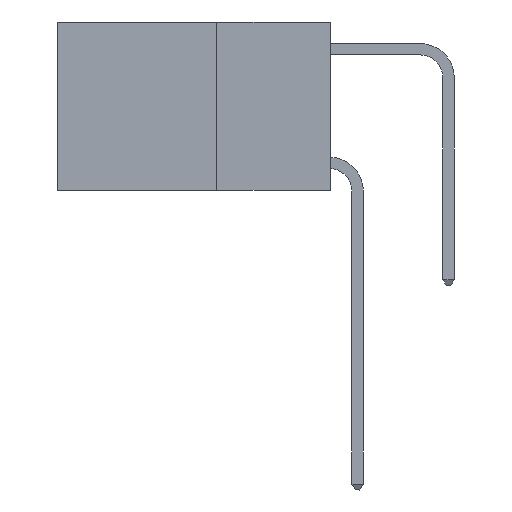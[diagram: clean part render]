
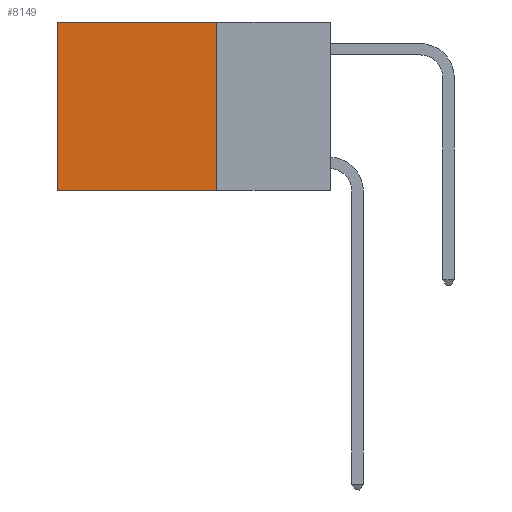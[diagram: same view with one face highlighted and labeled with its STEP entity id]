
A CAD part, left-side view. The second image highlights one B-rep face of the part: STEP entity #8149.
In plain terms, the highlighted planar face has unit normal (-1, 0, 0).
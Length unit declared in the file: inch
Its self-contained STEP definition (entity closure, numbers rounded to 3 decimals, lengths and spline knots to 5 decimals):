
#208 = CARTESIAN_POINT ( 'NONE',  ( 0.2625, 0.25, -0.37 ) ) ;
#336 = CARTESIAN_POINT ( 'NONE',  ( 0.2625, 0.25, 0. ) ) ;
#380 = EDGE_LOOP ( 'NONE', ( #4517, #14074, #3040, #14092 ) ) ;
#546 = DIRECTION ( 'NONE',  ( 0., 0., -1. ) ) ;
#625 = LINE ( 'NONE', #14130, #2360 ) ;
#1012 = VERTEX_POINT ( 'NONE', #6513 ) ;
#2041 = DIRECTION ( 'NONE',  ( 0., 1., 0. ) ) ;
#2360 = VECTOR ( 'NONE', #10369, 39.37008 ) ;
#3040 = ORIENTED_EDGE ( 'NONE', *, *, #4638, .F. ) ;
#3182 = VERTEX_POINT ( 'NONE', #15724 ) ;
#3628 = VECTOR ( 'NONE', #2041, 39.37008 ) ;
#4517 = ORIENTED_EDGE ( 'NONE', *, *, #12804, .T. ) ;
#4638 = EDGE_CURVE ( 'NONE', #3182, #1012, #11636, .T. ) ;
#5042 = LINE ( 'NONE', #208, #11948 ) ;
#5520 = DIRECTION ( 'NONE',  ( 1., 0., 0. ) ) ;
#6513 = CARTESIAN_POINT ( 'NONE',  ( 0.2625, 0.25, -0.37 ) ) ;
#6858 = CARTESIAN_POINT ( 'NONE',  ( 0.2625, 0.25, 0. ) ) ;
#6894 = LINE ( 'NONE', #336, #3628 ) ;
#7502 = DIRECTION ( 'NONE',  ( 0., 1., 0. ) ) ;
#7866 = VERTEX_POINT ( 'NONE', #15822 ) ;
#8149 = ADVANCED_FACE ( 'NONE', ( #13934 ), #11691, .F. ) ;
#8699 = EDGE_CURVE ( 'NONE', #3182, #7866, #6894, .T. ) ;
#8737 = VECTOR ( 'NONE', #546, 39.37008 ) ;
#9136 = CARTESIAN_POINT ( 'NONE',  ( 0.2625, 0.25, 0. ) ) ;
#10369 = DIRECTION ( 'NONE',  ( 0., 0., -1. ) ) ;
#11636 = LINE ( 'NONE', #6858, #8737 ) ;
#11691 = PLANE ( 'NONE',  #13895 ) ;
#11948 = VECTOR ( 'NONE', #7502, 39.37008 ) ;
#12030 = VERTEX_POINT ( 'NONE', #15561 ) ;
#12804 = EDGE_CURVE ( 'NONE', #7866, #12030, #625, .T. ) ;
#13895 = AXIS2_PLACEMENT_3D ( 'NONE', #9136, #5520, #14183 ) ;
#13934 = FACE_OUTER_BOUND ( 'NONE', #380, .T. ) ;
#13964 = EDGE_CURVE ( 'NONE', #1012, #12030, #5042, .T. ) ;
#14074 = ORIENTED_EDGE ( 'NONE', *, *, #13964, .F. ) ;
#14092 = ORIENTED_EDGE ( 'NONE', *, *, #8699, .T. ) ;
#14130 = CARTESIAN_POINT ( 'NONE',  ( 0.2625, 0.6, 0. ) ) ;
#14183 = DIRECTION ( 'NONE',  ( 0., 0., -1. ) ) ;
#15561 = CARTESIAN_POINT ( 'NONE',  ( 0.2625, 0.6, -0.37 ) ) ;
#15724 = CARTESIAN_POINT ( 'NONE',  ( 0.2625, 0.25, 0. ) ) ;
#15822 = CARTESIAN_POINT ( 'NONE',  ( 0.2625, 0.6, 0. ) ) ;
